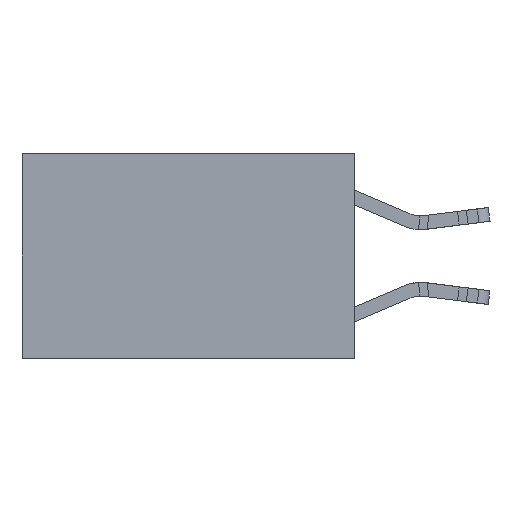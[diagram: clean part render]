
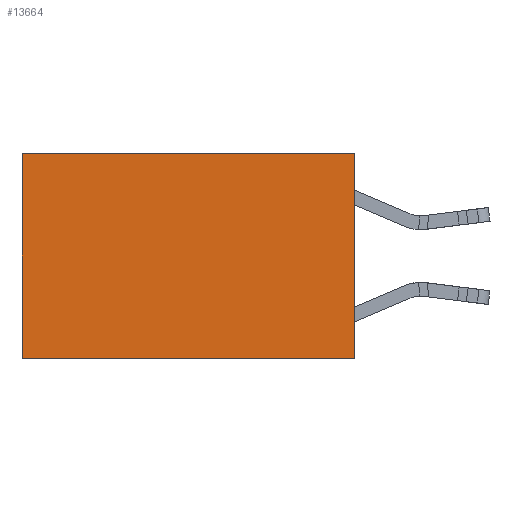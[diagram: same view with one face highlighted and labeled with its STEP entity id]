
A CAD part, left-side view. The second image highlights one B-rep face of the part: STEP entity #13664.
In plain terms, the highlighted planar face has unit normal (-1, 0, 0).
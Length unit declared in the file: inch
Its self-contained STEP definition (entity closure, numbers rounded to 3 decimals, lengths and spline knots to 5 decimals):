
#2 = ORIENTED_EDGE ( 'NONE', *, *, #14850, .F. ) ;
#120 = DIRECTION ( 'NONE',  ( 0., 1., 0. ) ) ;
#803 = VERTEX_POINT ( 'NONE', #25492 ) ;
#2344 = VECTOR ( 'NONE', #9418, 39.37008 ) ;
#3540 = EDGE_CURVE ( 'NONE', #8534, #15850, #8962, .T. ) ;
#5240 = CARTESIAN_POINT ( 'NONE',  ( 0.2625, 0., 0. ) ) ;
#5388 = EDGE_LOOP ( 'NONE', ( #26691, #24359, #2, #19862 ) ) ;
#5476 = VECTOR ( 'NONE', #120, 39.37008 ) ;
#5839 = CARTESIAN_POINT ( 'NONE',  ( 0.2625, 0., 0. ) ) ;
#6491 = LINE ( 'NONE', #25542, #10937 ) ;
#6555 = DIRECTION ( 'NONE',  ( 0., 0., -1. ) ) ;
#6856 = CARTESIAN_POINT ( 'NONE',  ( 0.2625, 0., 0. ) ) ;
#6902 = EDGE_CURVE ( 'NONE', #15850, #8855, #6491, .T. ) ;
#8342 = EDGE_CURVE ( 'NONE', #803, #8855, #9136, .T. ) ;
#8534 = VERTEX_POINT ( 'NONE', #5240 ) ;
#8855 = VERTEX_POINT ( 'NONE', #18715 ) ;
#8962 = LINE ( 'NONE', #9277, #2344 ) ;
#9136 = LINE ( 'NONE', #14234, #5476 ) ;
#9277 = CARTESIAN_POINT ( 'NONE',  ( 0.2625, 0., 0. ) ) ;
#9418 = DIRECTION ( 'NONE',  ( 0., 1., 0. ) ) ;
#10032 = LINE ( 'NONE', #5839, #27313 ) ;
#10937 = VECTOR ( 'NONE', #14228, 39.37008 ) ;
#13664 = ADVANCED_FACE ( 'NONE', ( #18202 ), #25300, .F. ) ;
#13899 = AXIS2_PLACEMENT_3D ( 'NONE', #6856, #16166, #6555 ) ;
#14228 = DIRECTION ( 'NONE',  ( 0., 0., -1. ) ) ;
#14234 = CARTESIAN_POINT ( 'NONE',  ( 0.2625, 0., -0.37 ) ) ;
#14850 = EDGE_CURVE ( 'NONE', #8534, #803, #10032, .T. ) ;
#15289 = DIRECTION ( 'NONE',  ( 0., 0., -1. ) ) ;
#15850 = VERTEX_POINT ( 'NONE', #22311 ) ;
#16166 = DIRECTION ( 'NONE',  ( 1., 0., 0. ) ) ;
#18202 = FACE_OUTER_BOUND ( 'NONE', #5388, .T. ) ;
#18715 = CARTESIAN_POINT ( 'NONE',  ( 0.2625, 0.6, -0.37 ) ) ;
#19862 = ORIENTED_EDGE ( 'NONE', *, *, #3540, .T. ) ;
#22311 = CARTESIAN_POINT ( 'NONE',  ( 0.2625, 0.6, 0. ) ) ;
#24359 = ORIENTED_EDGE ( 'NONE', *, *, #8342, .F. ) ;
#25300 = PLANE ( 'NONE',  #13899 ) ;
#25492 = CARTESIAN_POINT ( 'NONE',  ( 0.2625, 0., -0.37 ) ) ;
#25542 = CARTESIAN_POINT ( 'NONE',  ( 0.2625, 0.6, 0. ) ) ;
#26691 = ORIENTED_EDGE ( 'NONE', *, *, #6902, .T. ) ;
#27313 = VECTOR ( 'NONE', #15289, 39.37008 ) ;
